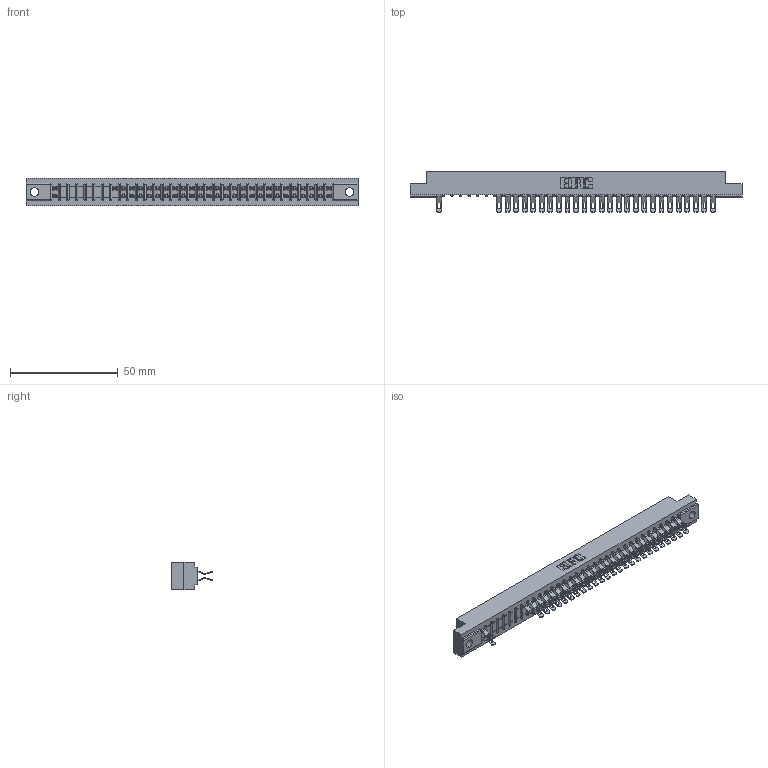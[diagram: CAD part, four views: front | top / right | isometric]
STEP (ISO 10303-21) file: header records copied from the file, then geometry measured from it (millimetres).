
FILE_DESCRIPTION (( 'STEP AP203' ), '1' );
FILE_NAME ('307-066-555-204.STEP', '2018-08-06T11:14:23', ( '' ), ( '' ), 'SwSTEP 2.0', 'SolidWorks 2016', '' );
FILE_SCHEMA (( 'CONFIG_CONTROL_DESIGN' ));
Length unit declared in the file: inch
Products named in the file (3): 307 Part_.156 Dia Mounting Holes; 307-290-001_555; 307-066-555-204
Assembly tree (54 placements, depth 2):
  307-066-555-204
    307 Part_.156 Dia Mounting Holes
    307-290-001_555  x53
Bounding box: 153.77 x 18.75 x 12.7 mm (x, y, z)
Volume: 16171.7 mm3; surface area: 19209.9 mm2
Topology: 54 solids, 54 shells, 3529 faces, 10368 edges, 6748 vertices
Faces by surface type: plane 1964, cylinder 1497, sphere 68
Entity records: 30995 total; most frequent: CARTESIAN_POINT 5138, ORIENTED_EDGE 5104, DIRECTION 5022, EDGE_CURVE 2552, VECTOR 1950, LINE 1950, VERTEX_POINT 1652, AXIS2_PLACEMENT_3D 1536
